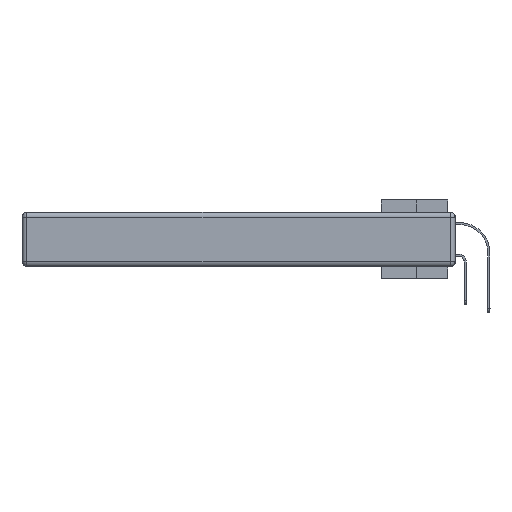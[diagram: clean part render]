
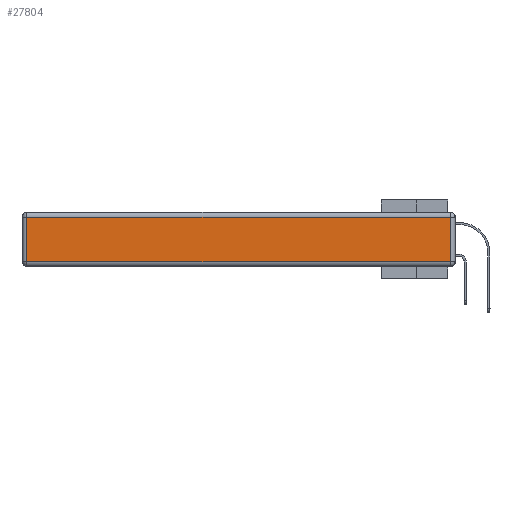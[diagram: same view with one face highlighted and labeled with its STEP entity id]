
A CAD part, left-side view. The second image highlights one B-rep face of the part: STEP entity #27804.
In plain terms, the highlighted planar face has unit normal (-1, 0, 0).
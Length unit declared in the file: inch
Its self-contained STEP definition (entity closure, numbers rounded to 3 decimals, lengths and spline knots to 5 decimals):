
#1329 = EDGE_CURVE ( 'NONE', #13135, #8897, #1978, .T. ) ;
#1978 = LINE ( 'NONE', #2700, #20974 ) ;
#2700 = CARTESIAN_POINT ( 'NONE',  ( 0., 0., -0.313 ) ) ;
#5285 = VERTEX_POINT ( 'NONE', #6075 ) ;
#6075 = CARTESIAN_POINT ( 'NONE',  ( 0., 0.03, -0.03 ) ) ;
#6213 = LINE ( 'NONE', #26553, #31681 ) ;
#6452 = CARTESIAN_POINT ( 'NONE',  ( 0., 2.72, -0.03 ) ) ;
#7182 = DIRECTION ( 'NONE',  ( 0., 1., 0. ) ) ;
#7931 = PLANE ( 'NONE',  #20036 ) ;
#8897 = VERTEX_POINT ( 'NONE', #27799 ) ;
#8996 = EDGE_CURVE ( 'NONE', #23462, #13135, #33485, .T. ) ;
#13135 = VERTEX_POINT ( 'NONE', #28860 ) ;
#14598 = ORIENTED_EDGE ( 'NONE', *, *, #24847, .T. ) ;
#15978 = LINE ( 'NONE', #24049, #26893 ) ;
#16188 = DIRECTION ( 'NONE',  ( -1., 0., 0. ) ) ;
#17946 = EDGE_LOOP ( 'NONE', ( #26352, #29010, #14598, #35725 ) ) ;
#19129 = DIRECTION ( 'NONE',  ( 0., 0., 1. ) ) ;
#20036 = AXIS2_PLACEMENT_3D ( 'NONE', #32899, #16188, #19129 ) ;
#20974 = VECTOR ( 'NONE', #30411, 39.37008 ) ;
#23462 = VERTEX_POINT ( 'NONE', #6452 ) ;
#24049 = CARTESIAN_POINT ( 'NONE',  ( 0., 2.75, -0.03 ) ) ;
#24381 = VECTOR ( 'NONE', #27431, 39.37008 ) ;
#24847 = EDGE_CURVE ( 'NONE', #5285, #23462, #15978, .T. ) ;
#25210 = CARTESIAN_POINT ( 'NONE',  ( 0., 2.72, -0.343 ) ) ;
#26352 = ORIENTED_EDGE ( 'NONE', *, *, #1329, .T. ) ;
#26553 = CARTESIAN_POINT ( 'NONE',  ( 0., 0.03, -0.343 ) ) ;
#26893 = VECTOR ( 'NONE', #7182, 39.37008 ) ;
#27431 = DIRECTION ( 'NONE',  ( 0., 0., -1. ) ) ;
#27799 = CARTESIAN_POINT ( 'NONE',  ( 0., 0.03, -0.313 ) ) ;
#27804 = ADVANCED_FACE ( 'NONE', ( #35636 ), #7931, .T. ) ;
#28775 = DIRECTION ( 'NONE',  ( 0., 0., 1. ) ) ;
#28860 = CARTESIAN_POINT ( 'NONE',  ( 0., 2.72, -0.313 ) ) ;
#29010 = ORIENTED_EDGE ( 'NONE', *, *, #32851, .T. ) ;
#30411 = DIRECTION ( 'NONE',  ( 0., -1., 0. ) ) ;
#31681 = VECTOR ( 'NONE', #28775, 39.37008 ) ;
#32851 = EDGE_CURVE ( 'NONE', #8897, #5285, #6213, .T. ) ;
#32899 = CARTESIAN_POINT ( 'NONE',  ( 0., 0., -0.343 ) ) ;
#33485 = LINE ( 'NONE', #25210, #24381 ) ;
#35636 = FACE_OUTER_BOUND ( 'NONE', #17946, .T. ) ;
#35725 = ORIENTED_EDGE ( 'NONE', *, *, #8996, .T. ) ;
